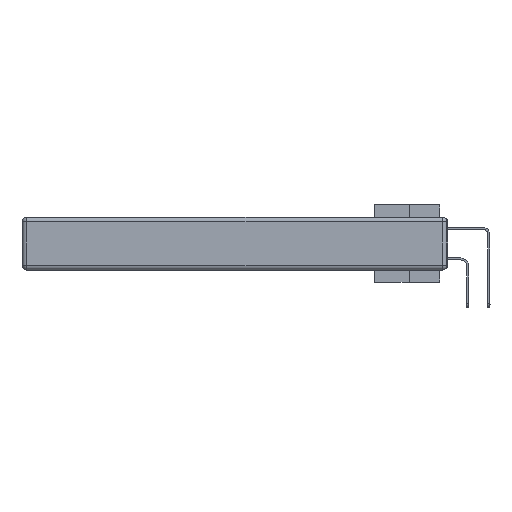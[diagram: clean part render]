
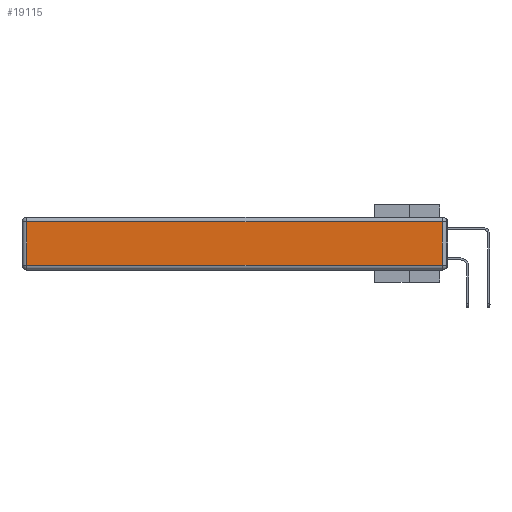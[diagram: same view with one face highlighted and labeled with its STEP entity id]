
A CAD part, left-side view. The second image highlights one B-rep face of the part: STEP entity #19115.
In plain terms, the highlighted planar face has unit normal (-1, 0, 0).
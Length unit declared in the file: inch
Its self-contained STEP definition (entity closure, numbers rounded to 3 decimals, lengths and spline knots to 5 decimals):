
#794 = CARTESIAN_POINT ( 'NONE',  ( 0., 0.03, -0.343 ) ) ;
#950 = DIRECTION ( 'NONE',  ( 0., 0., 1. ) ) ;
#2547 = FACE_OUTER_BOUND ( 'NONE', #25078, .T. ) ;
#3683 = EDGE_CURVE ( 'NONE', #23296, #27176, #5002, .T. ) ;
#4844 = CARTESIAN_POINT ( 'NONE',  ( 0., 2.72, -0.343 ) ) ;
#5002 = LINE ( 'NONE', #4844, #7290 ) ;
#5515 = LINE ( 'NONE', #794, #9103 ) ;
#6431 = CARTESIAN_POINT ( 'NONE',  ( 0., 0.03, -0.03 ) ) ;
#7290 = VECTOR ( 'NONE', #9518, 39.37008 ) ;
#9103 = VECTOR ( 'NONE', #950, 39.37008 ) ;
#9400 = ORIENTED_EDGE ( 'NONE', *, *, #3683, .T. ) ;
#9518 = DIRECTION ( 'NONE',  ( 0., 0., -1. ) ) ;
#10597 = VECTOR ( 'NONE', #13292, 39.37008 ) ;
#10798 = CARTESIAN_POINT ( 'NONE',  ( 0., 2.72, -0.03 ) ) ;
#11925 = CARTESIAN_POINT ( 'NONE',  ( 0., 0., -0.343 ) ) ;
#12910 = ORIENTED_EDGE ( 'NONE', *, *, #29203, .T. ) ;
#13292 = DIRECTION ( 'NONE',  ( 0., 1., 0. ) ) ;
#13542 = CARTESIAN_POINT ( 'NONE',  ( 0., 2.72, -0.313 ) ) ;
#15346 = EDGE_CURVE ( 'NONE', #21999, #23296, #25148, .T. ) ;
#16338 = DIRECTION ( 'NONE',  ( 0., -1., 0. ) ) ;
#16643 = CARTESIAN_POINT ( 'NONE',  ( 0., 0., -0.313 ) ) ;
#17932 = EDGE_CURVE ( 'NONE', #19037, #21999, #5515, .T. ) ;
#18480 = CARTESIAN_POINT ( 'NONE',  ( 0., 0.03, -0.313 ) ) ;
#19037 = VERTEX_POINT ( 'NONE', #18480 ) ;
#19115 = ADVANCED_FACE ( 'NONE', ( #2547 ), #23774, .T. ) ;
#19242 = DIRECTION ( 'NONE',  ( -1., 0., 0. ) ) ;
#20100 = AXIS2_PLACEMENT_3D ( 'NONE', #11925, #19242, #21594 ) ;
#21594 = DIRECTION ( 'NONE',  ( 0., 0., 1. ) ) ;
#21999 = VERTEX_POINT ( 'NONE', #6431 ) ;
#22054 = LINE ( 'NONE', #16643, #29308 ) ;
#23296 = VERTEX_POINT ( 'NONE', #10798 ) ;
#23774 = PLANE ( 'NONE',  #20100 ) ;
#25078 = EDGE_LOOP ( 'NONE', ( #12910, #25555, #28834, #9400 ) ) ;
#25148 = LINE ( 'NONE', #29836, #10597 ) ;
#25555 = ORIENTED_EDGE ( 'NONE', *, *, #17932, .T. ) ;
#27176 = VERTEX_POINT ( 'NONE', #13542 ) ;
#28834 = ORIENTED_EDGE ( 'NONE', *, *, #15346, .T. ) ;
#29203 = EDGE_CURVE ( 'NONE', #27176, #19037, #22054, .T. ) ;
#29308 = VECTOR ( 'NONE', #16338, 39.37008 ) ;
#29836 = CARTESIAN_POINT ( 'NONE',  ( 0., 2.75, -0.03 ) ) ;
